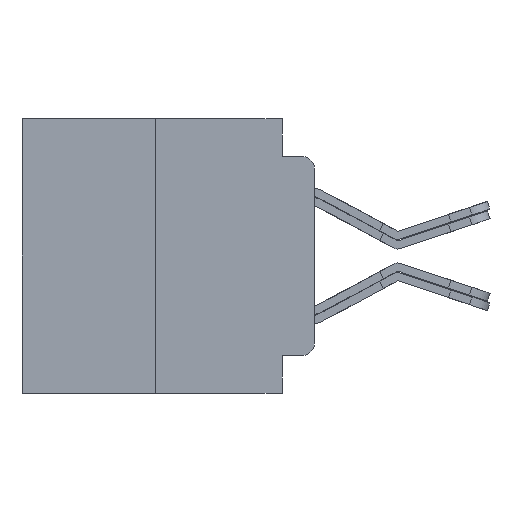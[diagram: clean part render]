
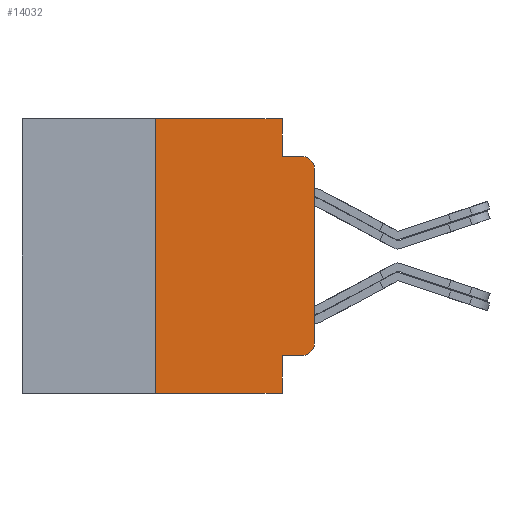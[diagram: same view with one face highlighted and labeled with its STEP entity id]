
A CAD part, left-side view. The second image highlights one B-rep face of the part: STEP entity #14032.
In plain terms, the highlighted planar face has unit normal (-1, 0, 0).
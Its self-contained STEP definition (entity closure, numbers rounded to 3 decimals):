
#569 = CARTESIAN_POINT ( 'NONE',  ( -75.603, 0.508, -3.467 ) ) ;
#1131 = VERTEX_POINT ( 'NONE', #1192 ) ;
#1192 = CARTESIAN_POINT ( 'NONE',  ( -75.603, 1.295, 3.975 ) ) ;
#1988 = FACE_OUTER_BOUND ( 'NONE', #22519, .T. ) ;
#2355 = VERTEX_POINT ( 'NONE', #2859 ) ;
#2466 = VECTOR ( 'NONE', #24169, 1000. ) ;
#2859 = CARTESIAN_POINT ( 'NONE',  ( -75.603, 6.35, -5.486 ) ) ;
#3094 = CARTESIAN_POINT ( 'NONE',  ( -75.603, 11.684, 5.486 ) ) ;
#3252 = VERTEX_POINT ( 'NONE', #26697 ) ;
#3253 = ORIENTED_EDGE ( 'NONE', *, *, #18603, .F. ) ;
#3455 = CARTESIAN_POINT ( 'NONE',  ( -75.603, 0.508, -3.975 ) ) ;
#3815 = ORIENTED_EDGE ( 'NONE', *, *, #19846, .T. ) ;
#3947 = VERTEX_POINT ( 'NONE', #4459 ) ;
#4000 = EDGE_CURVE ( 'NONE', #23293, #11973, #6887, .T. ) ;
#4368 = DIRECTION ( 'NONE',  ( 1., 0., 0. ) ) ;
#4459 = CARTESIAN_POINT ( 'NONE',  ( -75.603, 0., 3.467 ) ) ;
#4534 = EDGE_CURVE ( 'NONE', #2355, #3252, #15311, .T. ) ;
#4584 = EDGE_CURVE ( 'NONE', #11973, #3947, #13872, .T. ) ;
#4692 = CARTESIAN_POINT ( 'NONE',  ( -75.603, 1.295, -3.975 ) ) ;
#5621 = CARTESIAN_POINT ( 'NONE',  ( -75.603, 1.295, 0. ) ) ;
#6158 = DIRECTION ( 'NONE',  ( -1., 0., 0. ) ) ;
#6740 = LINE ( 'NONE', #10450, #2466 ) ;
#6822 = ORIENTED_EDGE ( 'NONE', *, *, #15910, .F. ) ;
#6887 = CIRCLE ( 'NONE', #28827, 0.508 ) ;
#6923 = ORIENTED_EDGE ( 'NONE', *, *, #22237, .F. ) ;
#7989 = VECTOR ( 'NONE', #12861, 1000. ) ;
#9778 = DIRECTION ( 'NONE',  ( 0., -1., 0. ) ) ;
#10175 = ORIENTED_EDGE ( 'NONE', *, *, #21883, .T. ) ;
#10320 = LINE ( 'NONE', #23379, #16271 ) ;
#10343 = ORIENTED_EDGE ( 'NONE', *, *, #13388, .F. ) ;
#10385 = CARTESIAN_POINT ( 'NONE',  ( -75.603, 1.295, 3.975 ) ) ;
#10450 = CARTESIAN_POINT ( 'NONE',  ( -75.603, 1.295, 0. ) ) ;
#10465 = LINE ( 'NONE', #4692, #27290 ) ;
#10860 = EDGE_CURVE ( 'NONE', #21867, #3252, #6740, .T. ) ;
#11760 = VECTOR ( 'NONE', #9778, 1000. ) ;
#11928 = CARTESIAN_POINT ( 'NONE',  ( -75.603, 1.295, 5.486 ) ) ;
#11973 = VERTEX_POINT ( 'NONE', #25747 ) ;
#12536 = CARTESIAN_POINT ( 'NONE',  ( -75.603, 0., 5.486 ) ) ;
#12621 = VECTOR ( 'NONE', #28644, 1000. ) ;
#12861 = DIRECTION ( 'NONE',  ( 0., -1., 0. ) ) ;
#13388 = EDGE_CURVE ( 'NONE', #18838, #15965, #14741, .T. ) ;
#13872 = LINE ( 'NONE', #12536, #27896 ) ;
#14032 = ADVANCED_FACE ( 'NONE', ( #1988 ), #26360, .F. ) ;
#14183 = DIRECTION ( 'NONE',  ( 0., 0., 1. ) ) ;
#14658 = AXIS2_PLACEMENT_3D ( 'NONE', #3094, #4368, #23473 ) ;
#14741 = LINE ( 'NONE', #28535, #12621 ) ;
#14959 = AXIS2_PLACEMENT_3D ( 'NONE', #19621, #6158, #23987 ) ;
#15016 = ORIENTED_EDGE ( 'NONE', *, *, #10860, .F. ) ;
#15311 = LINE ( 'NONE', #23295, #11760 ) ;
#15390 = LINE ( 'NONE', #10385, #7989 ) ;
#15910 = EDGE_CURVE ( 'NONE', #2355, #18838, #10320, .T. ) ;
#15965 = VERTEX_POINT ( 'NONE', #11928 ) ;
#16271 = VECTOR ( 'NONE', #14183, 1000. ) ;
#18298 = CARTESIAN_POINT ( 'NONE',  ( -75.603, 0.508, 3.975 ) ) ;
#18326 = CARTESIAN_POINT ( 'NONE',  ( -75.603, 1.295, -3.975 ) ) ;
#18376 = DIRECTION ( 'NONE',  ( -1., 0., 0. ) ) ;
#18603 = EDGE_CURVE ( 'NONE', #15965, #1131, #22615, .T. ) ;
#18838 = VERTEX_POINT ( 'NONE', #22025 ) ;
#19621 = CARTESIAN_POINT ( 'NONE',  ( -75.603, 0.508, 3.467 ) ) ;
#19846 = EDGE_CURVE ( 'NONE', #3947, #25020, #25297, .T. ) ;
#20607 = DIRECTION ( 'NONE',  ( 0., -1., 0. ) ) ;
#20823 = DIRECTION ( 'NONE',  ( 0., 0., -1. ) ) ;
#21867 = VERTEX_POINT ( 'NONE', #18326 ) ;
#21883 = EDGE_CURVE ( 'NONE', #21867, #23293, #10465, .T. ) ;
#22025 = CARTESIAN_POINT ( 'NONE',  ( -75.603, 6.35, 5.486 ) ) ;
#22237 = EDGE_CURVE ( 'NONE', #1131, #25020, #15390, .T. ) ;
#22519 = EDGE_LOOP ( 'NONE', ( #10175, #24067, #26882, #3815, #6923, #3253, #10343, #6822, #25876, #15016 ) ) ;
#22615 = LINE ( 'NONE', #5621, #25734 ) ;
#23293 = VERTEX_POINT ( 'NONE', #3455 ) ;
#23295 = CARTESIAN_POINT ( 'NONE',  ( -75.603, 11.684, -5.486 ) ) ;
#23379 = CARTESIAN_POINT ( 'NONE',  ( -75.603, 6.35, -5.486 ) ) ;
#23473 = DIRECTION ( 'NONE',  ( 0., 0., -1. ) ) ;
#23945 = DIRECTION ( 'NONE',  ( 0., 0., -1. ) ) ;
#23987 = DIRECTION ( 'NONE',  ( 0., 0., -1. ) ) ;
#24067 = ORIENTED_EDGE ( 'NONE', *, *, #4000, .T. ) ;
#24169 = DIRECTION ( 'NONE',  ( 0., 0., -1. ) ) ;
#25020 = VERTEX_POINT ( 'NONE', #18298 ) ;
#25297 = CIRCLE ( 'NONE', #14959, 0.508 ) ;
#25734 = VECTOR ( 'NONE', #23945, 1000. ) ;
#25747 = CARTESIAN_POINT ( 'NONE',  ( -75.603, 0., -3.467 ) ) ;
#25876 = ORIENTED_EDGE ( 'NONE', *, *, #4534, .T. ) ;
#26044 = DIRECTION ( 'NONE',  ( 0., 0., 1. ) ) ;
#26360 = PLANE ( 'NONE',  #14658 ) ;
#26697 = CARTESIAN_POINT ( 'NONE',  ( -75.603, 1.295, -5.486 ) ) ;
#26882 = ORIENTED_EDGE ( 'NONE', *, *, #4584, .T. ) ;
#27290 = VECTOR ( 'NONE', #20607, 1000. ) ;
#27896 = VECTOR ( 'NONE', #26044, 1000. ) ;
#28535 = CARTESIAN_POINT ( 'NONE',  ( -75.603, 11.684, 5.486 ) ) ;
#28644 = DIRECTION ( 'NONE',  ( 0., -1., 0. ) ) ;
#28827 = AXIS2_PLACEMENT_3D ( 'NONE', #569, #18376, #20823 ) ;
